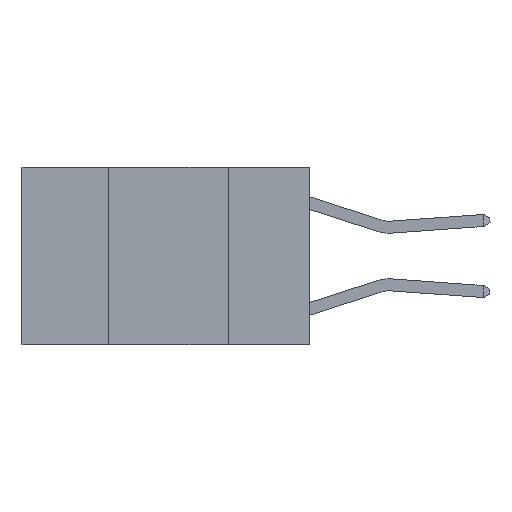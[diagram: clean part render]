
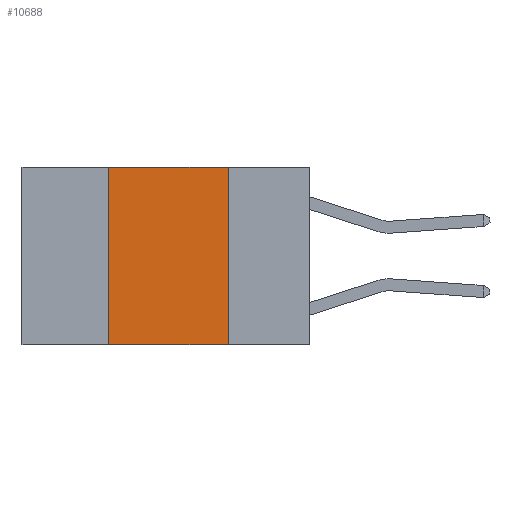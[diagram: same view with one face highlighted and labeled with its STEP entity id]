
A CAD part, left-side view. The second image highlights one B-rep face of the part: STEP entity #10688.
In plain terms, the highlighted planar face has unit normal (-1, 0, 0).
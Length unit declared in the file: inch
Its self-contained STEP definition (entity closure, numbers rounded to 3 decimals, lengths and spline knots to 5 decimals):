
#69 = CARTESIAN_POINT ( 'NONE',  ( 0., 0.42, 0. ) ) ;
#457 = ORIENTED_EDGE ( 'NONE', *, *, #6264, .F. ) ;
#1910 = AXIS2_PLACEMENT_3D ( 'NONE', #9719, #22561, #11547 ) ;
#2535 = CARTESIAN_POINT ( 'NONE',  ( 0., 0.17, 0. ) ) ;
#2959 = DIRECTION ( 'NONE',  ( 0., 0., -1. ) ) ;
#3053 = EDGE_CURVE ( 'NONE', #8380, #12522, #23992, .T. ) ;
#3945 = VECTOR ( 'NONE', #19591, 39.37008 ) ;
#4125 = ORIENTED_EDGE ( 'NONE', *, *, #23612, .T. ) ;
#4488 = CARTESIAN_POINT ( 'NONE',  ( 0., 0.17, -0.37 ) ) ;
#4549 = LINE ( 'NONE', #17747, #3945 ) ;
#4857 = CARTESIAN_POINT ( 'NONE',  ( 0., 0.6, 0. ) ) ;
#5895 = EDGE_CURVE ( 'NONE', #6893, #8380, #8925, .T. ) ;
#6264 = EDGE_CURVE ( 'NONE', #16354, #6893, #20375, .T. ) ;
#6569 = CARTESIAN_POINT ( 'NONE',  ( 0., 0.42, -0.37 ) ) ;
#6893 = VERTEX_POINT ( 'NONE', #69 ) ;
#8380 = VERTEX_POINT ( 'NONE', #2535 ) ;
#8521 = EDGE_LOOP ( 'NONE', ( #15067, #23724, #457, #4125 ) ) ;
#8925 = LINE ( 'NONE', #4857, #23012 ) ;
#9647 = DIRECTION ( 'NONE',  ( 0., 0., 1. ) ) ;
#9719 = CARTESIAN_POINT ( 'NONE',  ( 0., 0.6, 0. ) ) ;
#10688 = ADVANCED_FACE ( 'NONE', ( #21976 ), #18753, .F. ) ;
#11547 = DIRECTION ( 'NONE',  ( 0., 0., -1. ) ) ;
#12522 = VERTEX_POINT ( 'NONE', #4488 ) ;
#15067 = ORIENTED_EDGE ( 'NONE', *, *, #3053, .F. ) ;
#15499 = VECTOR ( 'NONE', #9647, 39.37008 ) ;
#15893 = DIRECTION ( 'NONE',  ( 0., -1., 0. ) ) ;
#16354 = VERTEX_POINT ( 'NONE', #6569 ) ;
#17747 = CARTESIAN_POINT ( 'NONE',  ( 0., 0.6, -0.37 ) ) ;
#18753 = PLANE ( 'NONE',  #1910 ) ;
#18759 = CARTESIAN_POINT ( 'NONE',  ( 0., 0.42, 0. ) ) ;
#19591 = DIRECTION ( 'NONE',  ( 0., -1., 0. ) ) ;
#20375 = LINE ( 'NONE', #18759, #15499 ) ;
#21976 = FACE_OUTER_BOUND ( 'NONE', #8521, .T. ) ;
#22561 = DIRECTION ( 'NONE',  ( 1., 0., 0. ) ) ;
#23012 = VECTOR ( 'NONE', #15893, 39.37008 ) ;
#23211 = CARTESIAN_POINT ( 'NONE',  ( 0., 0.17, 0. ) ) ;
#23390 = VECTOR ( 'NONE', #2959, 39.37008 ) ;
#23612 = EDGE_CURVE ( 'NONE', #16354, #12522, #4549, .T. ) ;
#23724 = ORIENTED_EDGE ( 'NONE', *, *, #5895, .F. ) ;
#23992 = LINE ( 'NONE', #23211, #23390 ) ;
